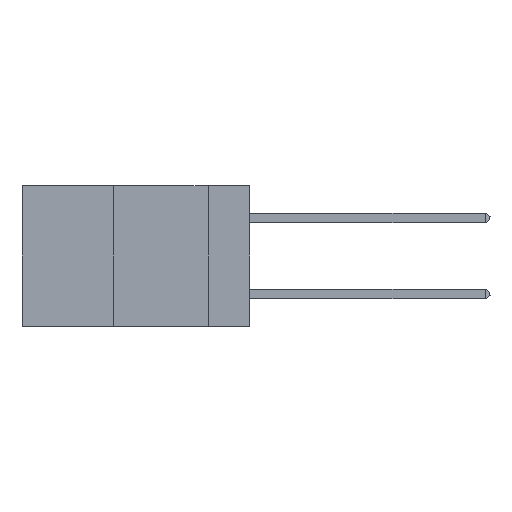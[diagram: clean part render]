
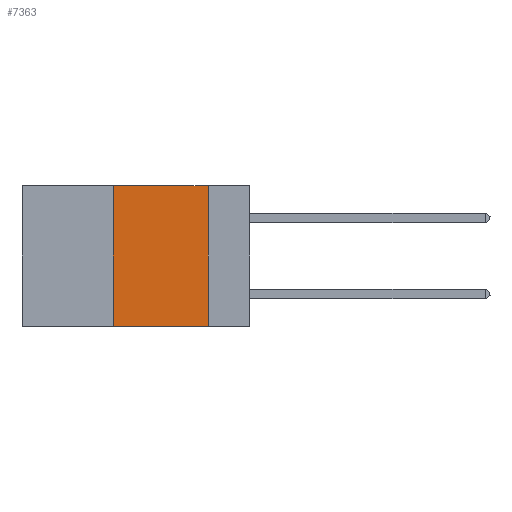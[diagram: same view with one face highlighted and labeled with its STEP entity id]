
A CAD part, left-side view. The second image highlights one B-rep face of the part: STEP entity #7363.
In plain terms, the highlighted planar face has unit normal (-1, 0, 0).
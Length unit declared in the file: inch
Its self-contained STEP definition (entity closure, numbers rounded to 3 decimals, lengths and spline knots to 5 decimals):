
#1606 = CARTESIAN_POINT ( 'NONE',  ( 0., 0.11, 0. ) ) ;
#1639 = DIRECTION ( 'NONE',  ( 0., 0., -1. ) ) ;
#1827 = VERTEX_POINT ( 'NONE', #1606 ) ;
#3488 = FACE_OUTER_BOUND ( 'NONE', #5914, .T. ) ;
#3785 = VECTOR ( 'NONE', #20327, 39.37008 ) ;
#3859 = VECTOR ( 'NONE', #15222, 39.37008 ) ;
#4090 = ORIENTED_EDGE ( 'NONE', *, *, #19475, .T. ) ;
#4955 = LINE ( 'NONE', #14409, #17172 ) ;
#5324 = ORIENTED_EDGE ( 'NONE', *, *, #15502, .F. ) ;
#5914 = EDGE_LOOP ( 'NONE', ( #8941, #8406, #5324, #4090 ) ) ;
#5969 = CARTESIAN_POINT ( 'NONE',  ( 0., 0.36, 0. ) ) ;
#7363 = ADVANCED_FACE ( 'NONE', ( #3488 ), #9837, .F. ) ;
#7672 = LINE ( 'NONE', #13386, #15626 ) ;
#8406 = ORIENTED_EDGE ( 'NONE', *, *, #17834, .F. ) ;
#8941 = ORIENTED_EDGE ( 'NONE', *, *, #13413, .F. ) ;
#9387 = CARTESIAN_POINT ( 'NONE',  ( 0., 0.6, -0.37 ) ) ;
#9687 = DIRECTION ( 'NONE',  ( 0., 0., 1. ) ) ;
#9837 = PLANE ( 'NONE',  #19780 ) ;
#10109 = CARTESIAN_POINT ( 'NONE',  ( 0., 0.11, -0.37 ) ) ;
#11397 = DIRECTION ( 'NONE',  ( 1., 0., 0. ) ) ;
#12073 = CARTESIAN_POINT ( 'NONE',  ( 0., 0.6, 0. ) ) ;
#12773 = VERTEX_POINT ( 'NONE', #14992 ) ;
#13386 = CARTESIAN_POINT ( 'NONE',  ( 0., 0.11, 0. ) ) ;
#13413 = EDGE_CURVE ( 'NONE', #1827, #15655, #7672, .T. ) ;
#14409 = CARTESIAN_POINT ( 'NONE',  ( 0., 0.36, 0. ) ) ;
#14968 = DIRECTION ( 'NONE',  ( 0., 0., -1. ) ) ;
#14992 = CARTESIAN_POINT ( 'NONE',  ( 0., 0.36, -0.37 ) ) ;
#15222 = DIRECTION ( 'NONE',  ( 0., -1., 0. ) ) ;
#15502 = EDGE_CURVE ( 'NONE', #12773, #16648, #4955, .T. ) ;
#15626 = VECTOR ( 'NONE', #14968, 39.37008 ) ;
#15655 = VERTEX_POINT ( 'NONE', #10109 ) ;
#16648 = VERTEX_POINT ( 'NONE', #5969 ) ;
#17172 = VECTOR ( 'NONE', #9687, 39.37008 ) ;
#17834 = EDGE_CURVE ( 'NONE', #16648, #1827, #20271, .T. ) ;
#19475 = EDGE_CURVE ( 'NONE', #12773, #15655, #19702, .T. ) ;
#19702 = LINE ( 'NONE', #9387, #3785 ) ;
#19780 = AXIS2_PLACEMENT_3D ( 'NONE', #20737, #11397, #1639 ) ;
#20271 = LINE ( 'NONE', #12073, #3859 ) ;
#20327 = DIRECTION ( 'NONE',  ( 0., -1., 0. ) ) ;
#20737 = CARTESIAN_POINT ( 'NONE',  ( 0., 0.6, 0. ) ) ;
